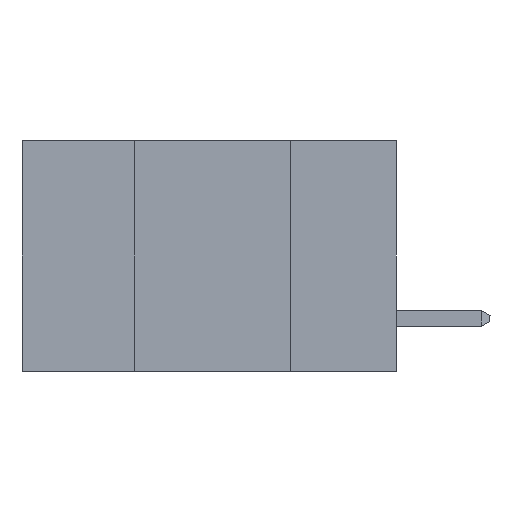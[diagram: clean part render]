
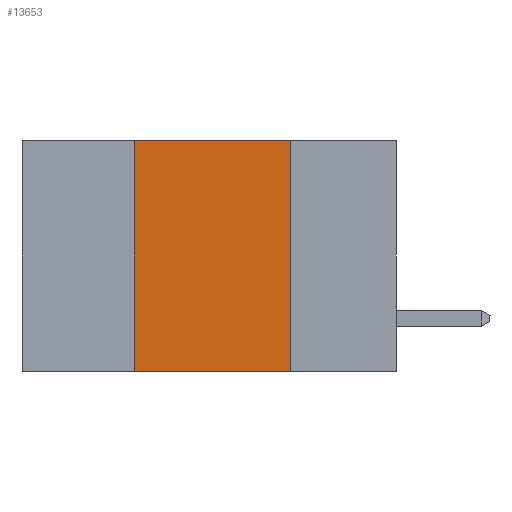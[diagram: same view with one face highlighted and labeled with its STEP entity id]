
A CAD part, left-side view. The second image highlights one B-rep face of the part: STEP entity #13653.
In plain terms, the highlighted planar face has unit normal (-1, 0, 0).
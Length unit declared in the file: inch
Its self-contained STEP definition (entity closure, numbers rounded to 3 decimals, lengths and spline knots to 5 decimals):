
#859 = LINE ( 'NONE', #2187, #5185 ) ;
#1169 = EDGE_CURVE ( 'NONE', #5748, #13236, #2693, .T. ) ;
#1693 = CARTESIAN_POINT ( 'NONE',  ( 0., 0.17, -0.37 ) ) ;
#2032 = DIRECTION ( 'NONE',  ( 0., -1., 0. ) ) ;
#2187 = CARTESIAN_POINT ( 'NONE',  ( 0., 0.6, -0.37 ) ) ;
#2251 = FACE_OUTER_BOUND ( 'NONE', #3226, .T. ) ;
#2693 = LINE ( 'NONE', #11824, #8096 ) ;
#2918 = EDGE_CURVE ( 'NONE', #5128, #5748, #14164, .T. ) ;
#3179 = EDGE_CURVE ( 'NONE', #13236, #11349, #10257, .T. ) ;
#3226 = EDGE_LOOP ( 'NONE', ( #6041, #9763, #11884, #9545 ) ) ;
#3565 = DIRECTION ( 'NONE',  ( 0., 0., -1. ) ) ;
#3674 = DIRECTION ( 'NONE',  ( 0., 0., -1. ) ) ;
#3903 = VECTOR ( 'NONE', #3674, 39.37008 ) ;
#4767 = AXIS2_PLACEMENT_3D ( 'NONE', #8019, #11178, #3565 ) ;
#5128 = VERTEX_POINT ( 'NONE', #9643 ) ;
#5185 = VECTOR ( 'NONE', #2032, 39.37008 ) ;
#5748 = VERTEX_POINT ( 'NONE', #9770 ) ;
#6041 = ORIENTED_EDGE ( 'NONE', *, *, #3179, .F. ) ;
#6703 = PLANE ( 'NONE',  #4767 ) ;
#6935 = CARTESIAN_POINT ( 'NONE',  ( 0., 0.17, 0. ) ) ;
#7144 = DIRECTION ( 'NONE',  ( 0., -1., 0. ) ) ;
#8019 = CARTESIAN_POINT ( 'NONE',  ( 0., 0.6, 0. ) ) ;
#8096 = VECTOR ( 'NONE', #7144, 39.37008 ) ;
#9545 = ORIENTED_EDGE ( 'NONE', *, *, #9668, .T. ) ;
#9643 = CARTESIAN_POINT ( 'NONE',  ( 0., 0.42, -0.37 ) ) ;
#9668 = EDGE_CURVE ( 'NONE', #5128, #11349, #859, .T. ) ;
#9763 = ORIENTED_EDGE ( 'NONE', *, *, #1169, .F. ) ;
#9770 = CARTESIAN_POINT ( 'NONE',  ( 0., 0.42, 0. ) ) ;
#10257 = LINE ( 'NONE', #11507, #3903 ) ;
#11178 = DIRECTION ( 'NONE',  ( 1., 0., 0. ) ) ;
#11349 = VERTEX_POINT ( 'NONE', #1693 ) ;
#11507 = CARTESIAN_POINT ( 'NONE',  ( 0., 0.17, -0.37 ) ) ;
#11824 = CARTESIAN_POINT ( 'NONE',  ( 0., 0.6, 0. ) ) ;
#11884 = ORIENTED_EDGE ( 'NONE', *, *, #2918, .F. ) ;
#12914 = DIRECTION ( 'NONE',  ( 0., 0., 1. ) ) ;
#13023 = VECTOR ( 'NONE', #12914, 39.37008 ) ;
#13236 = VERTEX_POINT ( 'NONE', #6935 ) ;
#13653 = ADVANCED_FACE ( 'NONE', ( #2251 ), #6703, .F. ) ;
#14096 = CARTESIAN_POINT ( 'NONE',  ( 0., 0.42, -0.37 ) ) ;
#14164 = LINE ( 'NONE', #14096, #13023 ) ;
